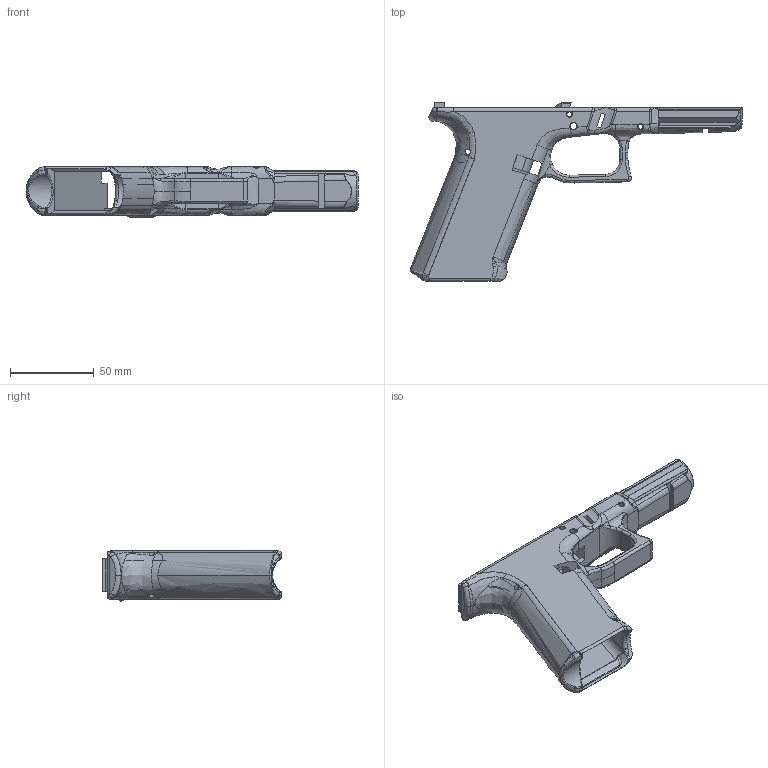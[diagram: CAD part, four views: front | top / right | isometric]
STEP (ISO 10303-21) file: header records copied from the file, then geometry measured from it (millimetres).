
FILE_DESCRIPTION(/* description */ (''),/* implementation_level */ '2;1');
FILE_NAME(/* name */ 'FMDA DD17.2 V1.4 Frame.stp',/* time_stamp */ '2020-12-27T21:57:02-06:00',/* author */ ('johne'),/* organization */ (''),/* preprocessor_version */ 'ST-DEVELOPER v18',/* originating_system */ 'Autodesk Inventor 2020',/* authorisation */ '');
FILE_SCHEMA (('AUTOMOTIVE_DESIGN { 1 0 10303 214 3 1 1 }'));
Products named in the file (1): Part66 no thumbs
Bounding box: 197.63 x 106.5 x 29.84 mm (x, y, z)
Volume: 86049.5 mm3; surface area: 47066.5 mm2
Topology: 1 solids, 3 shells, 664 faces, 1873 edges, 1183 vertices
Faces by surface type: bspline 295, plane 184, cylinder 136, torus 21, sphere 16, cone 12
Full cylindrical faces by diameter (mm): 2 x1, 3 x4, 3.2 x2, 4 x2
Entity records: 51698 total; most frequent: CARTESIAN_POINT 36412, ORIENTED_EDGE 3728, DIRECTION 2500, EDGE_CURVE 1864, VERTEX_POINT 1186, AXIS2_PLACEMENT_3D 911, LINE 678, VECTOR 678
